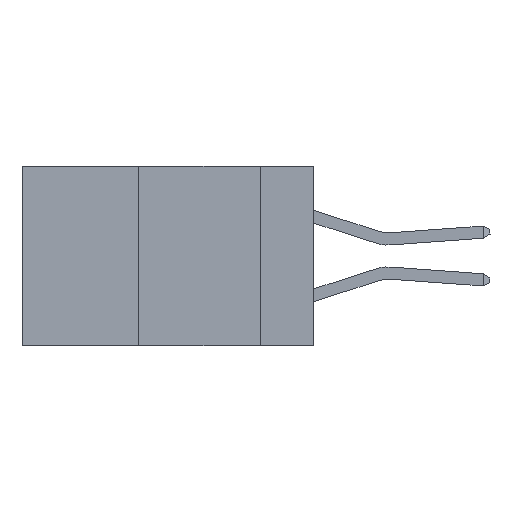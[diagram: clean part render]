
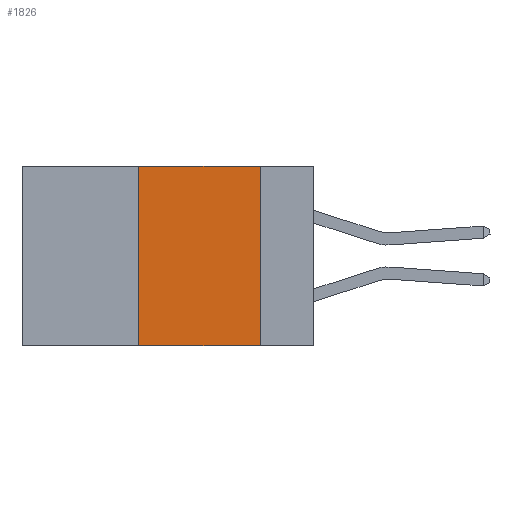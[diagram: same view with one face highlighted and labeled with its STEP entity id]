
A CAD part, left-side view. The second image highlights one B-rep face of the part: STEP entity #1826.
In plain terms, the highlighted planar face has unit normal (-1, 0, 0).
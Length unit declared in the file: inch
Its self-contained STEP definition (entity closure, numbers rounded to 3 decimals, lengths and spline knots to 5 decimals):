
#156 = DIRECTION ( 'NONE',  ( 1., 0., 0. ) ) ;
#251 = EDGE_CURVE ( 'NONE', #6113, #3608, #6521, .T. ) ;
#308 = CARTESIAN_POINT ( 'NONE',  ( 0., 0.11, 0. ) ) ;
#423 = CARTESIAN_POINT ( 'NONE',  ( 0., 0.11, 0. ) ) ;
#537 = AXIS2_PLACEMENT_3D ( 'NONE', #8280, #156, #1931 ) ;
#731 = CARTESIAN_POINT ( 'NONE',  ( 0., 0.11, -0.37 ) ) ;
#1826 = ADVANCED_FACE ( 'NONE', ( #7128 ), #7195, .F. ) ;
#1931 = DIRECTION ( 'NONE',  ( 0., 0., -1. ) ) ;
#2888 = LINE ( 'NONE', #5904, #6993 ) ;
#3204 = ORIENTED_EDGE ( 'NONE', *, *, #8502, .T. ) ;
#3608 = VERTEX_POINT ( 'NONE', #308 ) ;
#3623 = DIRECTION ( 'NONE',  ( 0., -1., 0. ) ) ;
#3964 = VERTEX_POINT ( 'NONE', #5082 ) ;
#4006 = CARTESIAN_POINT ( 'NONE',  ( 0., 0.6, 0. ) ) ;
#4216 = DIRECTION ( 'NONE',  ( 0., 0., 1. ) ) ;
#4558 = EDGE_LOOP ( 'NONE', ( #5934, #5044, #4580, #3204 ) ) ;
#4580 = ORIENTED_EDGE ( 'NONE', *, *, #9881, .F. ) ;
#5044 = ORIENTED_EDGE ( 'NONE', *, *, #251, .F. ) ;
#5082 = CARTESIAN_POINT ( 'NONE',  ( 0., 0.36, -0.37 ) ) ;
#5667 = VECTOR ( 'NONE', #4216, 39.37008 ) ;
#5904 = CARTESIAN_POINT ( 'NONE',  ( 0., 0.6, -0.37 ) ) ;
#5934 = ORIENTED_EDGE ( 'NONE', *, *, #9445, .F. ) ;
#6113 = VERTEX_POINT ( 'NONE', #9957 ) ;
#6521 = LINE ( 'NONE', #4006, #8259 ) ;
#6993 = VECTOR ( 'NONE', #9590, 39.37008 ) ;
#7128 = FACE_OUTER_BOUND ( 'NONE', #4558, .T. ) ;
#7195 = PLANE ( 'NONE',  #537 ) ;
#7232 = VECTOR ( 'NONE', #8442, 39.37008 ) ;
#8120 = CARTESIAN_POINT ( 'NONE',  ( 0., 0.36, 0. ) ) ;
#8259 = VECTOR ( 'NONE', #3623, 39.37008 ) ;
#8280 = CARTESIAN_POINT ( 'NONE',  ( 0., 0.6, 0. ) ) ;
#8442 = DIRECTION ( 'NONE',  ( 0., 0., -1. ) ) ;
#8502 = EDGE_CURVE ( 'NONE', #3964, #9964, #2888, .T. ) ;
#9105 = LINE ( 'NONE', #423, #7232 ) ;
#9445 = EDGE_CURVE ( 'NONE', #3608, #9964, #9105, .T. ) ;
#9590 = DIRECTION ( 'NONE',  ( 0., -1., 0. ) ) ;
#9616 = LINE ( 'NONE', #8120, #5667 ) ;
#9881 = EDGE_CURVE ( 'NONE', #3964, #6113, #9616, .T. ) ;
#9957 = CARTESIAN_POINT ( 'NONE',  ( 0., 0.36, 0. ) ) ;
#9964 = VERTEX_POINT ( 'NONE', #731 ) ;
